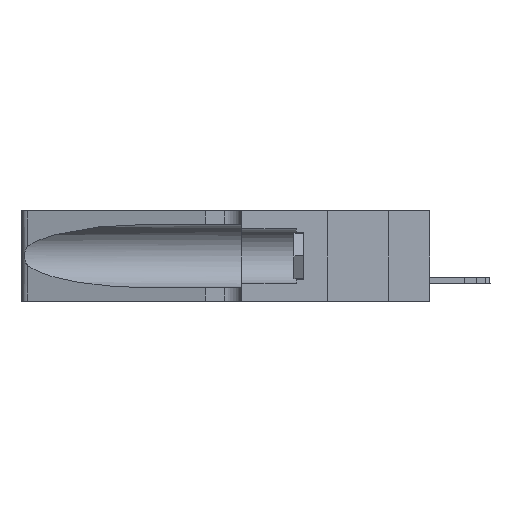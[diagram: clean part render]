
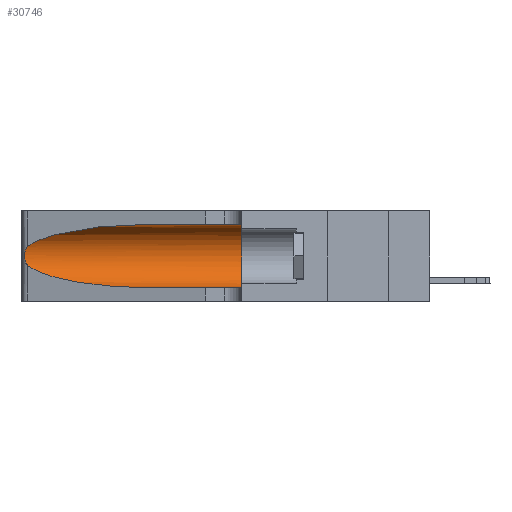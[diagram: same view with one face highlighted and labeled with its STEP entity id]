
A CAD part, left-side view. The second image highlights one B-rep face of the part: STEP entity #30746.
In plain terms, the highlighted cylindrical face has radius 3.308 mm (diameter 6.617 mm), a partial arc.
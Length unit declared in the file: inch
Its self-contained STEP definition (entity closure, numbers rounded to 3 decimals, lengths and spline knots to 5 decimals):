
#228 = CARTESIAN_POINT ( 'NONE',  ( 0.25487, 1.22718, 0.14631 ) ) ;
#385 = B_SPLINE_CURVE_WITH_KNOTS ( 'NONE', 3,
 ( #12216, #14958, #2868, #11654, #24831, #36881, #6020, #5760, #30687, #27933, #27523, #40152, #33584, #17956 ),
 .UNSPECIFIED., .F., .F.,
 ( 4, 2, 2, 2, 2, 2, 4 ),
 ( 0., 0.00027, 0.00053, 0.00107, 0.0016, 0.00187, 0.00214 ),
 .UNSPECIFIED. ) ;
#1421 = CARTESIAN_POINT ( 'NONE',  ( 0.1305, 0.72297, 0.31525 ) ) ;
#2203 = DIRECTION ( 'NONE',  ( 0., 1., 0. ) ) ;
#2314 = ORIENTED_EDGE ( 'NONE', *, *, #13733, .T. ) ;
#2472 = DIRECTION ( 'NONE',  ( 0., 0., 1. ) ) ;
#2868 = CARTESIAN_POINT ( 'NONE',  ( 0.25639, 1.23184, 0.21858 ) ) ;
#4465 = CARTESIAN_POINT ( 'NONE',  ( 0.1305, 1.61858, 0.185 ) ) ;
#5681 = EDGE_CURVE ( 'NONE', #27287, #25192, #6424, .T. ) ;
#5760 = CARTESIAN_POINT ( 'NONE',  ( 0.26075, 1.23896, 0.178 ) ) ;
#6020 = CARTESIAN_POINT ( 'NONE',  ( 0.26075, 1.23896, 0.19203 ) ) ;
#6424 =( BOUNDED_CURVE ( )  B_SPLINE_CURVE ( 3, ( #38495, #35872, #25871, #10643 ),
 .UNSPECIFIED., .F., .F. ) 
 B_SPLINE_CURVE_WITH_KNOTS ( ( 4, 4 ),
 ( 3.44316, 4.71239 ),
 .UNSPECIFIED. ) 
 CURVE ( )  GEOMETRIC_REPRESENTATION_ITEM ( )  RATIONAL_B_SPLINE_CURVE ( ( 1., 0.87, 0.87, 1. ) ) 
 REPRESENTATION_ITEM ( '' )  );
#6554 = ORIENTED_EDGE ( 'NONE', *, *, #22955, .F. ) ;
#7246 = VERTEX_POINT ( 'NONE', #10348 ) ;
#7256 = ORIENTED_EDGE ( 'NONE', *, *, #7650, .T. ) ;
#7650 = EDGE_CURVE ( 'NONE', #25192, #27950, #30589, .T. ) ;
#9000 = AXIS2_PLACEMENT_3D ( 'NONE', #30003, #2203, #2472 ) ;
#10348 = CARTESIAN_POINT ( 'NONE',  ( 0.25487, 1.22718, 0.22369 ) ) ;
#10643 = CARTESIAN_POINT ( 'NONE',  ( 0.1305, 0.72297, 0.05475 ) ) ;
#11654 = CARTESIAN_POINT ( 'NONE',  ( 0.25787, 1.23484, 0.2124 ) ) ;
#12216 = CARTESIAN_POINT ( 'NONE',  ( 0.25487, 1.22718, 0.22369 ) ) ;
#13689 = VECTOR ( 'NONE', #31265, 39.37008 ) ;
#13733 = EDGE_CURVE ( 'NONE', #36331, #7246, #28282, .T. ) ;
#14200 = AXIS2_PLACEMENT_3D ( 'NONE', #4465, #20086, #22987 ) ;
#14219 = EDGE_CURVE ( 'NONE', #7246, #27287, #385, .T. ) ;
#14422 = VERTEX_POINT ( 'NONE', #16408 ) ;
#14445 = CARTESIAN_POINT ( 'NONE',  ( 0.1305, 1.61858, 0.31525 ) ) ;
#14667 = CYLINDRICAL_SURFACE ( 'NONE', #14200, 0.13025 ) ;
#14958 = CARTESIAN_POINT ( 'NONE',  ( 0.25555, 1.22994, 0.2215 ) ) ;
#16064 = CARTESIAN_POINT ( 'NONE',  ( 0.1305, 0.72297, 0.31525 ) ) ;
#16408 = CARTESIAN_POINT ( 'NONE',  ( 0.1305, 0.35, 0.31525 ) ) ;
#16571 = DIRECTION ( 'NONE',  ( 0., -1., 0. ) ) ;
#17956 = CARTESIAN_POINT ( 'NONE',  ( 0.25487, 1.22718, 0.14631 ) ) ;
#19637 = CARTESIAN_POINT ( 'NONE',  ( 0.25487, 1.22718, 0.22369 ) ) ;
#20086 = DIRECTION ( 'NONE',  ( 0., -1., 0. ) ) ;
#20676 = EDGE_CURVE ( 'NONE', #36331, #14422, #26418, .T. ) ;
#22028 = FACE_OUTER_BOUND ( 'NONE', #30227, .T. ) ;
#22108 = ORIENTED_EDGE ( 'NONE', *, *, #5681, .T. ) ;
#22519 = CARTESIAN_POINT ( 'NONE',  ( 0.2373, 1.15595, 0.28018 ) ) ;
#22955 = EDGE_CURVE ( 'NONE', #14422, #27950, #30179, .T. ) ;
#22987 = DIRECTION ( 'NONE',  ( 0., 0., -1. ) ) ;
#24831 = CARTESIAN_POINT ( 'NONE',  ( 0.25854, 1.2359, 0.20912 ) ) ;
#25192 = VERTEX_POINT ( 'NONE', #33359 ) ;
#25637 = ORIENTED_EDGE ( 'NONE', *, *, #20676, .F. ) ;
#25871 = CARTESIAN_POINT ( 'NONE',  ( 0.18966, 0.96281, 0.05475 ) ) ;
#26418 = LINE ( 'NONE', #14445, #13689 ) ;
#27287 = VERTEX_POINT ( 'NONE', #228 ) ;
#27523 = CARTESIAN_POINT ( 'NONE',  ( 0.25789, 1.23486, 0.15765 ) ) ;
#27933 = CARTESIAN_POINT ( 'NONE',  ( 0.25856, 1.23593, 0.16098 ) ) ;
#27950 = VERTEX_POINT ( 'NONE', #37953 ) ;
#28149 = VECTOR ( 'NONE', #16571, 39.37008 ) ;
#28282 =( BOUNDED_CURVE ( )  B_SPLINE_CURVE ( 3, ( #16064, #38141, #22519, #19637 ),
 .UNSPECIFIED., .F., .T. ) 
 B_SPLINE_CURVE_WITH_KNOTS ( ( 4, 4 ),
 ( 1.5708, 2.84003 ),
 .UNSPECIFIED. ) 
 CURVE ( )  GEOMETRIC_REPRESENTATION_ITEM ( )  RATIONAL_B_SPLINE_CURVE ( ( 1., 0.87, 0.87, 1. ) ) 
 REPRESENTATION_ITEM ( '' )  );
#30003 = CARTESIAN_POINT ( 'NONE',  ( 0.1305, 0.35, 0.185 ) ) ;
#30179 = CIRCLE ( 'NONE', #9000, 0.13025 ) ;
#30227 = EDGE_LOOP ( 'NONE', ( #2314, #37299, #22108, #7256, #6554, #25637 ) ) ;
#30589 = LINE ( 'NONE', #31929, #28149 ) ;
#30687 = CARTESIAN_POINT ( 'NONE',  ( 0.26017, 1.23833, 0.17102 ) ) ;
#30746 = ADVANCED_FACE ( 'NONE', ( #22028 ), #14667, .F. ) ;
#31265 = DIRECTION ( 'NONE',  ( 0., -1., 0. ) ) ;
#31929 = CARTESIAN_POINT ( 'NONE',  ( 0.1305, 1.61858, 0.05475 ) ) ;
#33359 = CARTESIAN_POINT ( 'NONE',  ( 0.1305, 0.72297, 0.05475 ) ) ;
#33584 = CARTESIAN_POINT ( 'NONE',  ( 0.25555, 1.22993, 0.14849 ) ) ;
#35872 = CARTESIAN_POINT ( 'NONE',  ( 0.2373, 1.15595, 0.08982 ) ) ;
#36331 = VERTEX_POINT ( 'NONE', #1421 ) ;
#36881 = CARTESIAN_POINT ( 'NONE',  ( 0.26018, 1.23835, 0.19895 ) ) ;
#37299 = ORIENTED_EDGE ( 'NONE', *, *, #14219, .T. ) ;
#37953 = CARTESIAN_POINT ( 'NONE',  ( 0.1305, 0.35, 0.05475 ) ) ;
#38141 = CARTESIAN_POINT ( 'NONE',  ( 0.18966, 0.96281, 0.31525 ) ) ;
#38495 = CARTESIAN_POINT ( 'NONE',  ( 0.25487, 1.22718, 0.14631 ) ) ;
#40152 = CARTESIAN_POINT ( 'NONE',  ( 0.25639, 1.23186, 0.15144 ) ) ;
